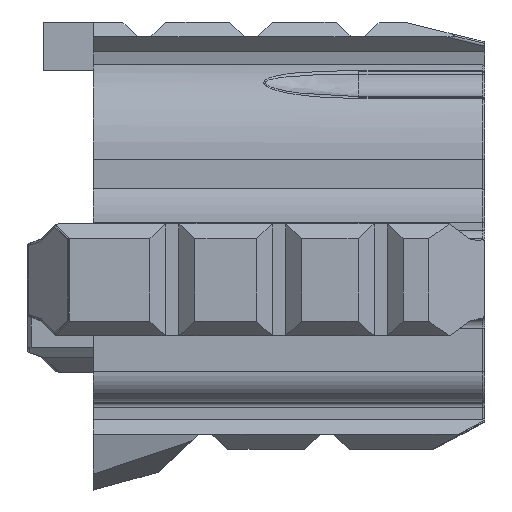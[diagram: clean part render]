
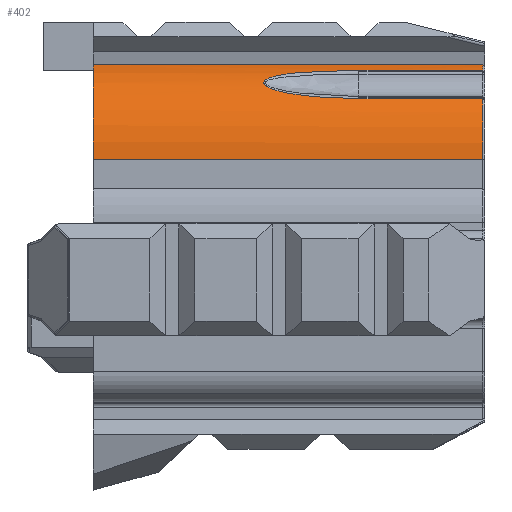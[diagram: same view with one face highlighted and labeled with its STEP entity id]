
A CAD part, top view. The second image highlights one B-rep face of the part: STEP entity #402.
In plain terms, the highlighted cylindrical face has radius 20.1 mm (diameter 40.2 mm), a partial arc.
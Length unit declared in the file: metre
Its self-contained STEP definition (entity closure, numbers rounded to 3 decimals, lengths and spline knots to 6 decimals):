
#402=ADVANCED_FACE('5:2526',(#1358),#1359,.T.);
#1358=FACE_OUTER_BOUND('',#3551,.T.);
#1359=CYLINDRICAL_SURFACE('',#3552,0.0201);
#3551=EDGE_LOOP('',(#7001,#7002,#7003,#7004,#7005,#7006,#7007,#7008));
#3552=AXIS2_PLACEMENT_3D('',#7009,#7010,#7011);
#7001=ORIENTED_EDGE('',*,*,#10105,.F.);
#7002=ORIENTED_EDGE('',*,*,#9296,.F.);
#7003=ORIENTED_EDGE('',*,*,#10124,.F.);
#7004=ORIENTED_EDGE('',*,*,#9292,.F.);
#7005=ORIENTED_EDGE('',*,*,#10110,.F.);
#7006=ORIENTED_EDGE('',*,*,#10125,.F.);
#7007=ORIENTED_EDGE('',*,*,#10126,.T.);
#7008=ORIENTED_EDGE('',*,*,#10117,.F.);
#7009=CARTESIAN_POINT('',(-0.012072,0.047361,0.001));
#7010=DIRECTION('',(-1.0,0.0,0.));
#7011=DIRECTION('',(0.,0.,-1.0));
#9292=EDGE_CURVE('5:5403',#11195,#11197,#11198,.T.);
#9296=EDGE_CURVE('5:5394',#11203,#11205,#11206,.T.);
#10105=EDGE_CURVE('5:5349',#11205,#12528,#12532,.T.);
#10110=EDGE_CURVE('5:5373',#12537,#11195,#12539,.T.);
#10117=EDGE_CURVE('5:5385',#12528,#12549,#12550,.T.);
#10124=EDGE_CURVE('5:5409',#11197,#11203,#12559,.T.);
#10125=EDGE_CURVE('5:5412',#12560,#12537,#12561,.T.);
#10126=EDGE_CURVE('5:3423',#12560,#12549,#12562,.T.);
#11195=VERTEX_POINT('',#14026);
#11197=VERTEX_POINT('',#14028);
#11198=LINE('',#14029,#14030);
#11203=VERTEX_POINT('',#14036);
#11205=VERTEX_POINT('',#14038);
#11206=LINE('',#14039,#14040);
#12528=VERTEX_POINT('',#17763);
#12532=CIRCLE('',#17770,0.0201);
#12537=VERTEX_POINT('',#17776);
#12539=CIRCLE('',#17781,0.0201);
#12549=VERTEX_POINT('',#17795);
#12550=LINE('',#17796,#17797);
#12559=B_SPLINE_CURVE_WITH_KNOTS('',3,(#17809,#17810,#17811,#17812,#17813,#17814,#17815,#17816,#17817,#17818,#17819,#17820,#17821,#17822,#17823,#17824,#17825,#17826,#17827),.UNSPECIFIED.,.F.,.F.,(4,1,1,1,1,1,1,1,1,1,1,1,1,1,1,1,4),(-3.974023,-3.406305,-3.122447,-2.980517,-2.838588,-2.554729,-2.27087,-2.176251,-2.081631,-2.034321,-1.987011,-1.892392,-1.703153,-1.608533,-1.513913,-1.135435,0.0),.UNSPECIFIED.);
#12560=VERTEX_POINT('',#17828);
#12561=LINE('',#17829,#17830);
#12562=CIRCLE('',#17831,0.0201);
#14026=CARTESIAN_POINT('',(0.0883,0.064924,0.010776));
#14028=CARTESIAN_POINT('',(0.06396,0.064924,0.010776));
#14029=CARTESIAN_POINT('',(0.190555,0.064924,0.010776));
#14030=VECTOR('',#19474,0.024339);
#14036=CARTESIAN_POINT('',(0.06396,0.059295,0.017174));
#14038=CARTESIAN_POINT('',(0.0883,0.059295,0.017174));
#14039=CARTESIAN_POINT('',(0.190555,0.059295,0.017174));
#14040=VECTOR('',#19482,0.024339);
#17763=CARTESIAN_POINT('',(0.0883,0.047361,0.0211));
#17770=AXIS2_PLACEMENT_3D('',#20299,#20300,#20301);
#17776=CARTESIAN_POINT('',(0.0883,0.065991,0.008545));
#17781=AXIS2_PLACEMENT_3D('',#20309,#20310,#20311);
#17795=CARTESIAN_POINT('',(0.011678,0.047361,0.0211));
#17796=CARTESIAN_POINT('',(-0.012072,0.047361,0.0211));
#17797=VECTOR('',#20322,0.076622);
#17809=CARTESIAN_POINT('',(0.06396,0.064924,0.010776));
#17810=CARTESIAN_POINT('',(0.062068,0.064924,0.010776));
#17811=CARTESIAN_POINT('',(0.059228,0.06488,0.010855));
#17812=CARTESIAN_POINT('',(0.055931,0.064737,0.011106));
#17813=CARTESIAN_POINT('',(0.054049,0.064619,0.011305));
#17814=CARTESIAN_POINT('',(0.052173,0.064474,0.011546));
#17815=CARTESIAN_POINT('',(0.049862,0.064227,0.01194));
#17816=CARTESIAN_POINT('',(0.047724,0.06386,0.01249));
#17817=CARTESIAN_POINT('',(0.046315,0.063423,0.013087));
#17818=CARTESIAN_POINT('',(0.045675,0.063116,0.013486));
#17819=CARTESIAN_POINT('',(0.045302,0.062776,0.013902));
#17820=CARTESIAN_POINT('',(0.045137,0.062339,0.014412));
#17821=CARTESIAN_POINT('',(0.045726,0.061611,0.015192));
#17822=CARTESIAN_POINT('',(0.046878,0.061167,0.01561));
#17823=CARTESIAN_POINT('',(0.048041,0.060807,0.015942));
#17824=CARTESIAN_POINT('',(0.049861,0.060363,0.016333));
#17825=CARTESIAN_POINT('',(0.05512,0.059523,0.01702));
#17826=CARTESIAN_POINT('',(0.060176,0.059295,0.017174));
#17827=CARTESIAN_POINT('',(0.06396,0.059295,0.017174));
#17828=CARTESIAN_POINT('',(0.011678,0.065991,0.008545));
#17829=CARTESIAN_POINT('',(-0.012072,0.065991,0.008545));
#17830=VECTOR('',#20335,0.076622);
#17831=AXIS2_PLACEMENT_3D('',#20336,#20337,#20338);
#19474=DIRECTION('',(-1.0,0.0,0.));
#19482=DIRECTION('',(1.0,0.0,0.));
#20299=CARTESIAN_POINT('',(0.0883,0.047361,0.001));
#20300=DIRECTION('',(1.0,0.,0.));
#20301=DIRECTION('',(0.,0.,1.0));
#20309=CARTESIAN_POINT('',(0.0883,0.047361,0.001));
#20310=DIRECTION('',(1.0,0.,0.));
#20311=DIRECTION('',(0.,0.,1.0));
#20322=DIRECTION('',(-1.0,0.0,0.));
#20335=DIRECTION('',(1.0,0.0,0.));
#20336=CARTESIAN_POINT('',(0.011678,0.047361,0.001));
#20337=DIRECTION('',(1.0,0.,0.));
#20338=DIRECTION('',(0.,0.,-1.0));
